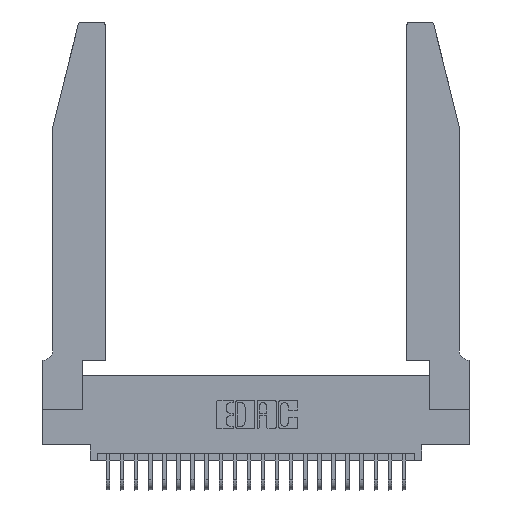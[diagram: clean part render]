
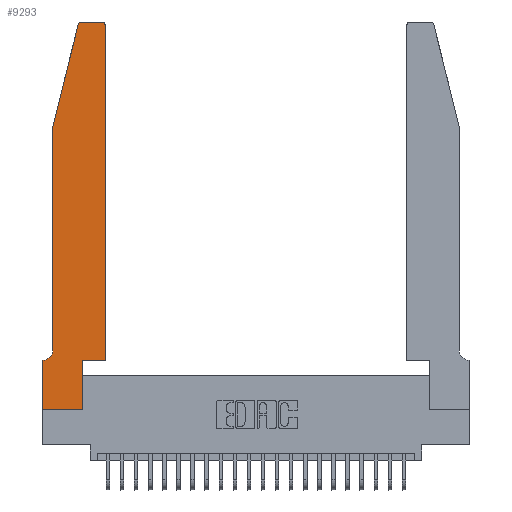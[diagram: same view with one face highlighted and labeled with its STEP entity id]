
A CAD part, top view. The second image highlights one B-rep face of the part: STEP entity #9293.
In plain terms, the highlighted planar face has unit normal (0, 0, 1).
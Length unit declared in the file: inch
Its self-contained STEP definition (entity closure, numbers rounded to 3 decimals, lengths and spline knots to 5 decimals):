
#289 = VECTOR ( 'NONE', #17480, 39.37008 ) ;
#432 = EDGE_CURVE ( 'NONE', #15082, #12678, #15510, .T. ) ;
#522 = EDGE_CURVE ( 'NONE', #694, #25591, #7825, .T. ) ;
#650 = LINE ( 'NONE', #25810, #5638 ) ;
#694 = VERTEX_POINT ( 'NONE', #2101 ) ;
#791 = EDGE_CURVE ( 'NONE', #6508, #3099, #12989, .T. ) ;
#803 = EDGE_CURVE ( 'NONE', #22008, #9666, #1878, .T. ) ;
#854 = CARTESIAN_POINT ( 'NONE',  ( 0.0055, 0.35, 0.37 ) ) ;
#1165 = EDGE_CURVE ( 'NONE', #12678, #4423, #10079, .T. ) ;
#1341 = ORIENTED_EDGE ( 'NONE', *, *, #12444, .T. ) ;
#1343 = DIRECTION ( 'NONE',  ( 0., -1., 0. ) ) ;
#1878 = LINE ( 'NONE', #24916, #22417 ) ;
#2101 = CARTESIAN_POINT ( 'NONE',  ( 0., 0.35, 0.37 ) ) ;
#3099 = VERTEX_POINT ( 'NONE', #9869 ) ;
#3311 = EDGE_LOOP ( 'NONE', ( #1341, #25492, #6063, #16711, #5602, #23807, #3951, #22981, #9021, #5940, #23395, #11842 ) ) ;
#3581 = PLANE ( 'NONE',  #22507 ) ;
#3951 = ORIENTED_EDGE ( 'NONE', *, *, #522, .T. ) ;
#4423 = VERTEX_POINT ( 'NONE', #9895 ) ;
#4546 = CARTESIAN_POINT ( 'NONE',  ( 0.4205, 2.75, 0.37 ) ) ;
#4816 = FACE_OUTER_BOUND ( 'NONE', #3311, .T. ) ;
#4982 = CARTESIAN_POINT ( 'NONE',  ( 0.4205, 2.72, 0.37 ) ) ;
#5602 = ORIENTED_EDGE ( 'NONE', *, *, #14622, .T. ) ;
#5623 = CARTESIAN_POINT ( 'NONE',  ( 0., 0.35, 0.37 ) ) ;
#5638 = VECTOR ( 'NONE', #1343, 39.37008 ) ;
#5710 = DIRECTION ( 'NONE',  ( 1., 0., 0. ) ) ;
#5940 = ORIENTED_EDGE ( 'NONE', *, *, #25725, .T. ) ;
#6063 = ORIENTED_EDGE ( 'NONE', *, *, #1165, .T. ) ;
#6088 = CARTESIAN_POINT ( 'NONE',  ( 0.0755, 0.35, 0.37 ) ) ;
#6508 = VERTEX_POINT ( 'NONE', #8952 ) ;
#6543 = CARTESIAN_POINT ( 'NONE',  ( 0., 0., 0.37 ) ) ;
#6935 = CARTESIAN_POINT ( 'NONE',  ( 0.0755, 2., 0.37 ) ) ;
#7082 = DIRECTION ( 'NONE',  ( 1., 0., 0. ) ) ;
#7196 = EDGE_CURVE ( 'NONE', #25591, #6508, #16872, .T. ) ;
#7825 = LINE ( 'NONE', #16027, #23979 ) ;
#8280 = CARTESIAN_POINT ( 'NONE',  ( 0.0055, 0.42, 0.37 ) ) ;
#8477 = DIRECTION ( 'NONE',  ( 1., 0., 0. ) ) ;
#8588 = DIRECTION ( 'NONE',  ( 0., 1., 0. ) ) ;
#8947 = VERTEX_POINT ( 'NONE', #4546 ) ;
#8952 = CARTESIAN_POINT ( 'NONE',  ( 0.2865, 0., 0.37 ) ) ;
#8964 = VECTOR ( 'NONE', #16449, 39.37008 ) ;
#9021 = ORIENTED_EDGE ( 'NONE', *, *, #791, .T. ) ;
#9293 = ADVANCED_FACE ( 'NONE', ( #4816 ), #3581, .T. ) ;
#9492 = CARTESIAN_POINT ( 'NONE',  ( 0.284, 2.72, 0.37 ) ) ;
#9666 = VERTEX_POINT ( 'NONE', #19143 ) ;
#9869 = CARTESIAN_POINT ( 'NONE',  ( 0.2865, 0.35, 0.37 ) ) ;
#9895 = CARTESIAN_POINT ( 'NONE',  ( 0.0755, 2., 0.37 ) ) ;
#10079 = LINE ( 'NONE', #6935, #26095 ) ;
#10378 = DIRECTION ( 'NONE',  ( -1., 0., 0. ) ) ;
#10657 = DIRECTION ( 'NONE',  ( 0., 1., 0. ) ) ;
#11182 = CARTESIAN_POINT ( 'NONE',  ( 0.4505, 0.35, 0.37 ) ) ;
#11419 = CIRCLE ( 'NONE', #17722, 0.03 ) ;
#11795 = CARTESIAN_POINT ( 'NONE',  ( 0.284, 2.75, 0.37 ) ) ;
#11842 = ORIENTED_EDGE ( 'NONE', *, *, #14330, .T. ) ;
#12085 = VERTEX_POINT ( 'NONE', #16015 ) ;
#12444 = EDGE_CURVE ( 'NONE', #8947, #15082, #16922, .T. ) ;
#12678 = VERTEX_POINT ( 'NONE', #23757 ) ;
#12989 = LINE ( 'NONE', #21284, #17721 ) ;
#13271 = DIRECTION ( 'NONE',  ( 1., 0., 0. ) ) ;
#14330 = EDGE_CURVE ( 'NONE', #9666, #8947, #11419, .T. ) ;
#14356 = CARTESIAN_POINT ( 'NONE',  ( 0.4505, 0.35, 0.37 ) ) ;
#14450 = LINE ( 'NONE', #6088, #8964 ) ;
#14622 = EDGE_CURVE ( 'NONE', #12085, #15474, #20593, .T. ) ;
#15082 = VERTEX_POINT ( 'NONE', #11795 ) ;
#15196 = DIRECTION ( 'NONE',  ( -1., 0., 0. ) ) ;
#15474 = VERTEX_POINT ( 'NONE', #854 ) ;
#15476 = CARTESIAN_POINT ( 'NONE',  ( 0., 0., 0.37 ) ) ;
#15510 = CIRCLE ( 'NONE', #19883, 0.03 ) ;
#15956 = LINE ( 'NONE', #11182, #25914 ) ;
#16015 = CARTESIAN_POINT ( 'NONE',  ( 0.0755, 0.42, 0.37 ) ) ;
#16027 = CARTESIAN_POINT ( 'NONE',  ( 0., 0., 0.37 ) ) ;
#16449 = DIRECTION ( 'NONE',  ( -1., 0., 0. ) ) ;
#16711 = ORIENTED_EDGE ( 'NONE', *, *, #21178, .T. ) ;
#16872 = LINE ( 'NONE', #15476, #289 ) ;
#16922 = LINE ( 'NONE', #21161, #22261 ) ;
#17207 = AXIS2_PLACEMENT_3D ( 'NONE', #8280, #22474, #10378 ) ;
#17335 = DIRECTION ( 'NONE',  ( 0., -1., 0. ) ) ;
#17480 = DIRECTION ( 'NONE',  ( 1., 0., 0. ) ) ;
#17629 = DIRECTION ( 'NONE',  ( -0.239, -0.971, 0. ) ) ;
#17721 = VECTOR ( 'NONE', #10657, 39.37008 ) ;
#17722 = AXIS2_PLACEMENT_3D ( 'NONE', #4982, #19334, #7082 ) ;
#18013 = DIRECTION ( 'NONE',  ( 0., 0., 1. ) ) ;
#19143 = CARTESIAN_POINT ( 'NONE',  ( 0.4505, 2.72, 0.37 ) ) ;
#19334 = DIRECTION ( 'NONE',  ( 0., 0., 1. ) ) ;
#19883 = AXIS2_PLACEMENT_3D ( 'NONE', #9492, #21029, #8477 ) ;
#20111 = EDGE_CURVE ( 'NONE', #15474, #694, #14450, .T. ) ;
#20593 = CIRCLE ( 'NONE', #17207, 0.07 ) ;
#21029 = DIRECTION ( 'NONE',  ( 0., 0., 1. ) ) ;
#21161 = CARTESIAN_POINT ( 'NONE',  ( 0.2605, 2.75, 0.37 ) ) ;
#21178 = EDGE_CURVE ( 'NONE', #4423, #12085, #650, .T. ) ;
#21284 = CARTESIAN_POINT ( 'NONE',  ( 0.2865, 0.35, 0.37 ) ) ;
#22008 = VERTEX_POINT ( 'NONE', #14356 ) ;
#22261 = VECTOR ( 'NONE', #15196, 39.37008 ) ;
#22417 = VECTOR ( 'NONE', #8588, 39.37008 ) ;
#22474 = DIRECTION ( 'NONE',  ( 0., 0., -1. ) ) ;
#22507 = AXIS2_PLACEMENT_3D ( 'NONE', #5623, #18013, #5710 ) ;
#22981 = ORIENTED_EDGE ( 'NONE', *, *, #7196, .T. ) ;
#23395 = ORIENTED_EDGE ( 'NONE', *, *, #803, .T. ) ;
#23757 = CARTESIAN_POINT ( 'NONE',  ( 0.25487, 2.72718, 0.37 ) ) ;
#23807 = ORIENTED_EDGE ( 'NONE', *, *, #20111, .T. ) ;
#23979 = VECTOR ( 'NONE', #17335, 39.37008 ) ;
#24916 = CARTESIAN_POINT ( 'NONE',  ( 0.4505, 0.35, 0.37 ) ) ;
#25492 = ORIENTED_EDGE ( 'NONE', *, *, #432, .T. ) ;
#25591 = VERTEX_POINT ( 'NONE', #6543 ) ;
#25725 = EDGE_CURVE ( 'NONE', #3099, #22008, #15956, .T. ) ;
#25810 = CARTESIAN_POINT ( 'NONE',  ( 0.0755, 2., 0.37 ) ) ;
#25914 = VECTOR ( 'NONE', #13271, 39.37008 ) ;
#26095 = VECTOR ( 'NONE', #17629, 39.37008 ) ;
